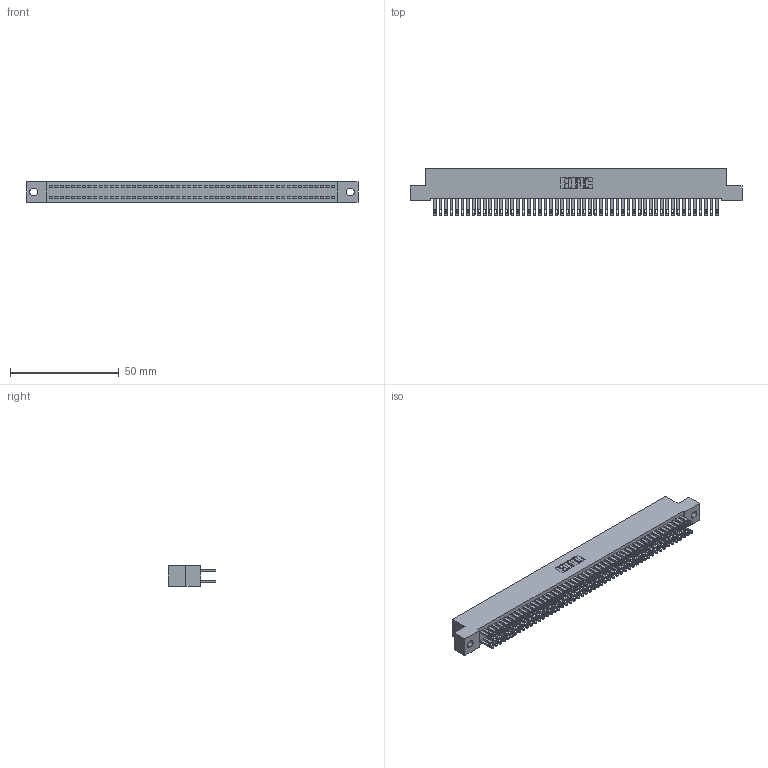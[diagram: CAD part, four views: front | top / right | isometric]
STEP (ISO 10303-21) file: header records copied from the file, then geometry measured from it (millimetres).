
FILE_DESCRIPTION (( 'STEP AP203' ), '1' );
FILE_NAME ('892-104-500-202.STEP', '2020-09-21T21:30:50', ( '' ), ( '' ), 'SwSTEP 2.0', 'SolidWorks 2020', '' );
FILE_SCHEMA (( 'CONFIG_CONTROL_DESIGN' ));
Length unit declared in the file: inch
Products named in the file (3): 842 Part_.128 Slot; 892-104-500-202; 345-292-001_345-293-100
Assembly tree (105 placements, depth 2):
  892-104-500-202
    842 Part_.128 Slot
    345-292-001_345-293-100  x104
Bounding box: 152.4 x 21.85 x 9.4 mm (x, y, z)
Volume: 14006.1 mm3; surface area: 23800.1 mm2
Topology: 105 solids, 105 shells, 5106 faces, 15599 edges, 10398 vertices
Faces by surface type: plane 3190, cylinder 1916
Entity records: 32093 total; most frequent: CARTESIAN_POINT 5306, ORIENTED_EDGE 5242, DIRECTION 4517, EDGE_CURVE 2621, LINE 2489, VECTOR 2489, VERTEX_POINT 1746, AXIS2_PLACEMENT_3D 1014
